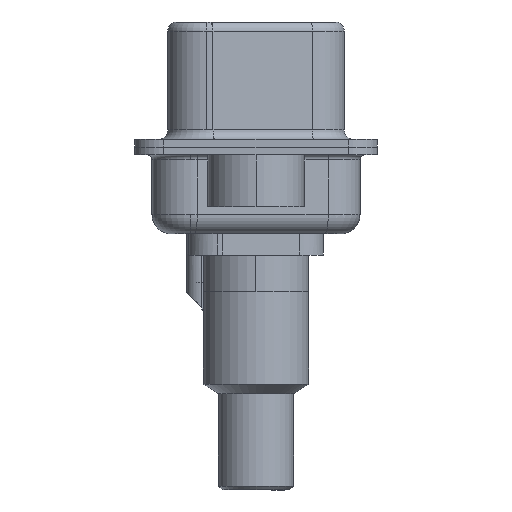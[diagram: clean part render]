
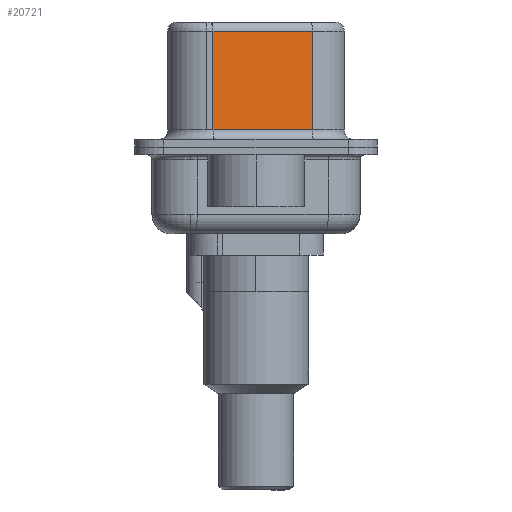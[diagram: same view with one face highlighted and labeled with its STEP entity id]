
A CAD part, left-side view. The second image highlights one B-rep face of the part: STEP entity #20721.
In plain terms, the highlighted planar face has unit normal (-0.985, -0.174, 0).
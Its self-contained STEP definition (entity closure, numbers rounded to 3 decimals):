
#773 = CARTESIAN_POINT ( 'NONE',  ( 3.67, 2.233, 0.9 ) ) ;
#1586 = CARTESIAN_POINT ( 'NONE',  ( 4.58, -2.927, 6.02 ) ) ;
#2084 = VECTOR ( 'NONE', #5021, 1000. ) ;
#2180 = VECTOR ( 'NONE', #4416, 1000. ) ;
#3608 = VERTEX_POINT ( 'NONE', #15592 ) ;
#3614 = ORIENTED_EDGE ( 'NONE', *, *, #23487, .F. ) ;
#4084 = VECTOR ( 'NONE', #10720, 1000. ) ;
#4416 = DIRECTION ( 'NONE',  ( 0., 0., -1. ) ) ;
#5021 = DIRECTION ( 'NONE',  ( 0.174, -0.985, 0. ) ) ;
#5111 = VERTEX_POINT ( 'NONE', #773 ) ;
#5932 = ORIENTED_EDGE ( 'NONE', *, *, #27963, .T. ) ;
#7141 = CARTESIAN_POINT ( 'NONE',  ( 4.58, -2.927, 0.9 ) ) ;
#7859 = CARTESIAN_POINT ( 'NONE',  ( 4.58, -2.927, 0.9 ) ) ;
#8055 = LINE ( 'NONE', #7141, #2084 ) ;
#8164 = LINE ( 'NONE', #13094, #2180 ) ;
#8592 = ORIENTED_EDGE ( 'NONE', *, *, #27774, .T. ) ;
#10720 = DIRECTION ( 'NONE',  ( -0.174, 0.985, 0. ) ) ;
#10923 = PLANE ( 'NONE',  #18753 ) ;
#11011 = DIRECTION ( 'NONE',  ( 0., 0., -1. ) ) ;
#13094 = CARTESIAN_POINT ( 'NONE',  ( 4.58, -2.927, 6.52 ) ) ;
#13109 = DIRECTION ( 'NONE',  ( -0.174, 0.985, 0. ) ) ;
#15100 = EDGE_CURVE ( 'NONE', #24042, #3608, #15108, .T. ) ;
#15108 = LINE ( 'NONE', #21764, #4084 ) ;
#15592 = CARTESIAN_POINT ( 'NONE',  ( 3.67, 2.233, 6.02 ) ) ;
#16555 = FACE_OUTER_BOUND ( 'NONE', #18978, .T. ) ;
#16621 = VECTOR ( 'NONE', #11011, 1000. ) ;
#18753 = AXIS2_PLACEMENT_3D ( 'NONE', #24112, #26314, #13109 ) ;
#18978 = EDGE_LOOP ( 'NONE', ( #3614, #25061, #8592, #5932 ) ) ;
#19801 = VERTEX_POINT ( 'NONE', #7859 ) ;
#20721 = ADVANCED_FACE ( 'NONE', ( #16555 ), #10923, .F. ) ;
#21764 = CARTESIAN_POINT ( 'NONE',  ( 4.58, -2.927, 6.02 ) ) ;
#23487 = EDGE_CURVE ( 'NONE', #24042, #19801, #8164, .T. ) ;
#24042 = VERTEX_POINT ( 'NONE', #1586 ) ;
#24112 = CARTESIAN_POINT ( 'NONE',  ( 4.58, -2.927, 6.52 ) ) ;
#25061 = ORIENTED_EDGE ( 'NONE', *, *, #15100, .T. ) ;
#26314 = DIRECTION ( 'NONE',  ( 0.985, 0.174, 0. ) ) ;
#26409 = CARTESIAN_POINT ( 'NONE',  ( 3.67, 2.233, 6.52 ) ) ;
#26972 = LINE ( 'NONE', #26409, #16621 ) ;
#27774 = EDGE_CURVE ( 'NONE', #3608, #5111, #26972, .T. ) ;
#27963 = EDGE_CURVE ( 'NONE', #5111, #19801, #8055, .T. ) ;
